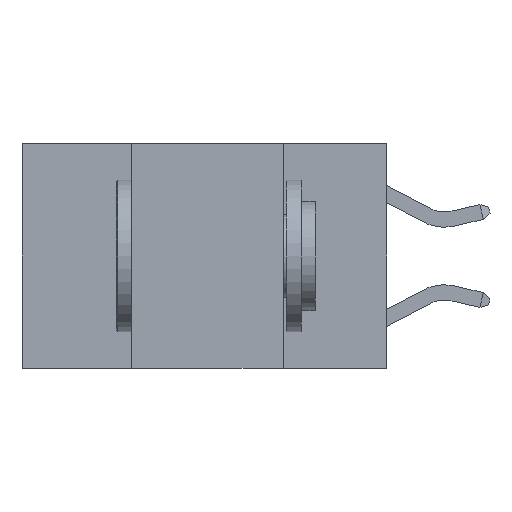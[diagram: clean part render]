
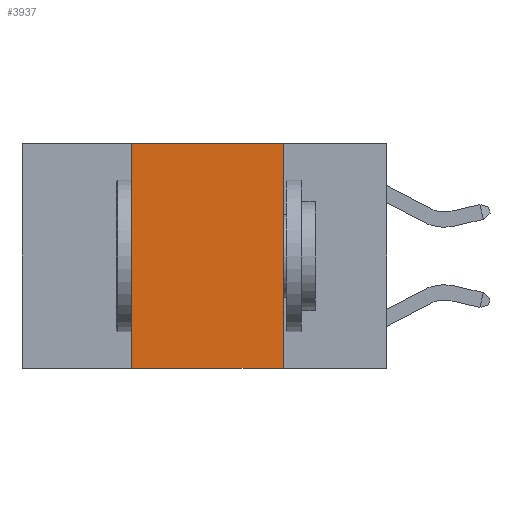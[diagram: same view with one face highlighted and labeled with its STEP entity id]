
A CAD part, left-side view. The second image highlights one B-rep face of the part: STEP entity #3937.
In plain terms, the highlighted planar face has unit normal (-1, 0, 0).
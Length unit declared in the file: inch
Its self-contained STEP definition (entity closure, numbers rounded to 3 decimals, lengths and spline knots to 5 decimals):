
#149 = VERTEX_POINT ( 'NONE', #11424 ) ;
#262 = VECTOR ( 'NONE', #6153, 39.37008 ) ;
#1020 = LINE ( 'NONE', #10304, #11005 ) ;
#1333 = ORIENTED_EDGE ( 'NONE', *, *, #9916, .F. ) ;
#1815 = DIRECTION ( 'NONE',  ( 0., 0., 1. ) ) ;
#1962 = CARTESIAN_POINT ( 'NONE',  ( 0., 0.6, 0. ) ) ;
#2067 = LINE ( 'NONE', #9162, #6280 ) ;
#2109 = VERTEX_POINT ( 'NONE', #3352 ) ;
#2857 = DIRECTION ( 'NONE',  ( 1., 0., 0. ) ) ;
#3352 = CARTESIAN_POINT ( 'NONE',  ( 0., 0.42, 0. ) ) ;
#3602 = FACE_OUTER_BOUND ( 'NONE', #6877, .T. ) ;
#3678 = DIRECTION ( 'NONE',  ( 0., -1., 0. ) ) ;
#3717 = ORIENTED_EDGE ( 'NONE', *, *, #3900, .F. ) ;
#3900 = EDGE_CURVE ( 'NONE', #2109, #149, #2067, .T. ) ;
#3937 = ADVANCED_FACE ( 'NONE', ( #3602 ), #7388, .F. ) ;
#3995 = ORIENTED_EDGE ( 'NONE', *, *, #6594, .T. ) ;
#5244 = CARTESIAN_POINT ( 'NONE',  ( 0., 0.6, -0.37 ) ) ;
#6153 = DIRECTION ( 'NONE',  ( 0., -1., 0. ) ) ;
#6280 = VECTOR ( 'NONE', #3678, 39.37008 ) ;
#6594 = EDGE_CURVE ( 'NONE', #7382, #8258, #6955, .T. ) ;
#6598 = CARTESIAN_POINT ( 'NONE',  ( 0., 0.42, -0.37 ) ) ;
#6626 = DIRECTION ( 'NONE',  ( 0., 0., -1. ) ) ;
#6877 = EDGE_LOOP ( 'NONE', ( #1333, #3717, #11040, #3995 ) ) ;
#6955 = LINE ( 'NONE', #5244, #262 ) ;
#7244 = CARTESIAN_POINT ( 'NONE',  ( 0., 0.42, 0. ) ) ;
#7382 = VERTEX_POINT ( 'NONE', #6598 ) ;
#7388 = PLANE ( 'NONE',  #9920 ) ;
#8258 = VERTEX_POINT ( 'NONE', #9762 ) ;
#9162 = CARTESIAN_POINT ( 'NONE',  ( 0., 0.6, 0. ) ) ;
#9240 = DIRECTION ( 'NONE',  ( 0., 0., -1. ) ) ;
#9687 = EDGE_CURVE ( 'NONE', #7382, #2109, #10282, .T. ) ;
#9762 = CARTESIAN_POINT ( 'NONE',  ( 0., 0.17, -0.37 ) ) ;
#9916 = EDGE_CURVE ( 'NONE', #149, #8258, #1020, .T. ) ;
#9920 = AXIS2_PLACEMENT_3D ( 'NONE', #1962, #2857, #9240 ) ;
#10282 = LINE ( 'NONE', #7244, #10580 ) ;
#10304 = CARTESIAN_POINT ( 'NONE',  ( 0., 0.17, 0. ) ) ;
#10580 = VECTOR ( 'NONE', #1815, 39.37008 ) ;
#11005 = VECTOR ( 'NONE', #6626, 39.37008 ) ;
#11040 = ORIENTED_EDGE ( 'NONE', *, *, #9687, .F. ) ;
#11424 = CARTESIAN_POINT ( 'NONE',  ( 0., 0.17, 0. ) ) ;
